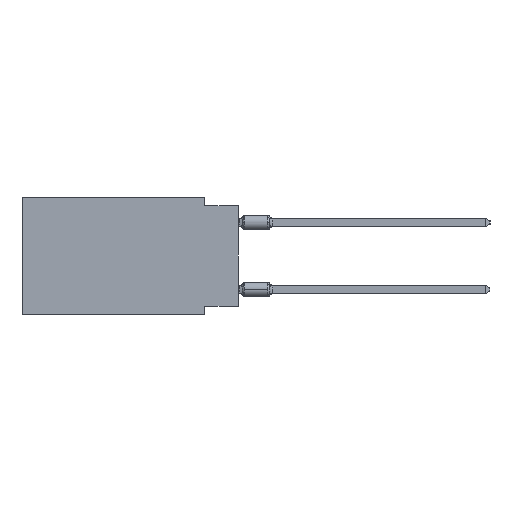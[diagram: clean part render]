
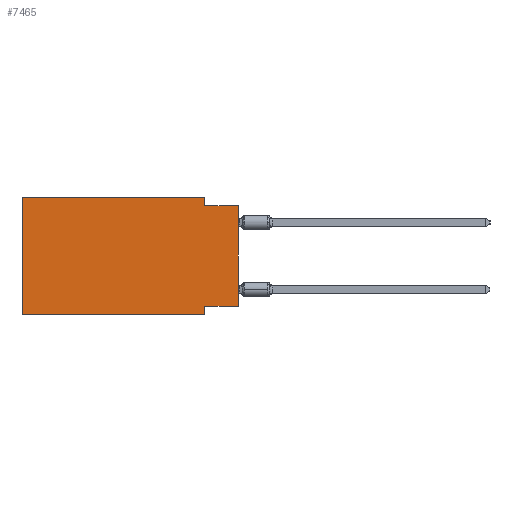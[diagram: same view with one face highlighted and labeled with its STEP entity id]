
A CAD part, left-side view. The second image highlights one B-rep face of the part: STEP entity #7465.
In plain terms, the highlighted planar face has unit normal (-1, 0, 0).
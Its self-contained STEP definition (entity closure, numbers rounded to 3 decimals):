
#809 = DIRECTION ( 'NONE',  ( 0., 0., -1. ) ) ;
#2652 = LINE ( 'NONE', #35970, #9058 ) ;
#2998 = VECTOR ( 'NONE', #25973, 1000. ) ;
#3244 = ORIENTED_EDGE ( 'NONE', *, *, #29201, .F. ) ;
#3809 = DIRECTION ( 'NONE',  ( 0., 1., 0. ) ) ;
#4959 = CARTESIAN_POINT ( 'NONE',  ( 0., 16.383, 0. ) ) ;
#5069 = FACE_OUTER_BOUND ( 'NONE', #7067, .T. ) ;
#5259 = LINE ( 'NONE', #28649, #10199 ) ;
#6622 = EDGE_CURVE ( 'NONE', #28197, #38506, #11860, .T. ) ;
#7067 = EDGE_LOOP ( 'NONE', ( #33655, #41532, #22445, #38807, #16646, #17941, #14594, #3244 ) ) ;
#7431 = AXIS2_PLACEMENT_3D ( 'NONE', #24636, #37595, #8459 ) ;
#7465 = ADVANCED_FACE ( 'NONE', ( #5069 ), #11648, .F. ) ;
#8037 = CARTESIAN_POINT ( 'NONE',  ( 0., 16.383, 0. ) ) ;
#8459 = DIRECTION ( 'NONE',  ( 0., 0., -1. ) ) ;
#8770 = EDGE_CURVE ( 'NONE', #38506, #9479, #41892, .T. ) ;
#9046 = DIRECTION ( 'NONE',  ( 0., -1., 0. ) ) ;
#9058 = VECTOR ( 'NONE', #38172, 1000. ) ;
#9479 = VERTEX_POINT ( 'NONE', #29926 ) ;
#10199 = VECTOR ( 'NONE', #15889, 1000. ) ;
#11470 = EDGE_CURVE ( 'NONE', #16207, #28123, #5259, .T. ) ;
#11648 = PLANE ( 'NONE',  #7431 ) ;
#11763 = VERTEX_POINT ( 'NONE', #16727 ) ;
#11860 = LINE ( 'NONE', #8037, #12814 ) ;
#12764 = CARTESIAN_POINT ( 'NONE',  ( 0., 16.383, 0. ) ) ;
#12814 = VECTOR ( 'NONE', #30595, 1000. ) ;
#12991 = LINE ( 'NONE', #22785, #2998 ) ;
#13105 = EDGE_CURVE ( 'NONE', #28197, #16300, #37562, .T. ) ;
#13923 = VECTOR ( 'NONE', #809, 1000. ) ;
#14243 = EDGE_CURVE ( 'NONE', #35062, #28123, #12991, .T. ) ;
#14594 = ORIENTED_EDGE ( 'NONE', *, *, #15758, .F. ) ;
#15758 = EDGE_CURVE ( 'NONE', #11763, #16300, #2652, .T. ) ;
#15889 = DIRECTION ( 'NONE',  ( 0., -1., 0. ) ) ;
#16207 = VERTEX_POINT ( 'NONE', #26573 ) ;
#16300 = VERTEX_POINT ( 'NONE', #36765 ) ;
#16646 = ORIENTED_EDGE ( 'NONE', *, *, #6622, .F. ) ;
#16727 = CARTESIAN_POINT ( 'NONE',  ( 0., 2.54, -8.255 ) ) ;
#17914 = VECTOR ( 'NONE', #9046, 1000. ) ;
#17941 = ORIENTED_EDGE ( 'NONE', *, *, #13105, .T. ) ;
#19251 = VECTOR ( 'NONE', #3809, 1000. ) ;
#22445 = ORIENTED_EDGE ( 'NONE', *, *, #23297, .F. ) ;
#22785 = CARTESIAN_POINT ( 'NONE',  ( 0., 0., 0. ) ) ;
#23297 = EDGE_CURVE ( 'NONE', #9479, #16207, #32961, .T. ) ;
#23388 = CARTESIAN_POINT ( 'NONE',  ( 0., 2.54, 0. ) ) ;
#24191 = VECTOR ( 'NONE', #25744, 1000. ) ;
#24636 = CARTESIAN_POINT ( 'NONE',  ( 0., 16.383, 0. ) ) ;
#25744 = DIRECTION ( 'NONE',  ( 0., -1., 0. ) ) ;
#25973 = DIRECTION ( 'NONE',  ( 0., 0., 1. ) ) ;
#26468 = CARTESIAN_POINT ( 'NONE',  ( 0., 0., -0.635 ) ) ;
#26573 = CARTESIAN_POINT ( 'NONE',  ( 0., 2.54, -0.635 ) ) ;
#28123 = VERTEX_POINT ( 'NONE', #26468 ) ;
#28197 = VERTEX_POINT ( 'NONE', #37088 ) ;
#28649 = CARTESIAN_POINT ( 'NONE',  ( 0., 0., -0.635 ) ) ;
#29201 = EDGE_CURVE ( 'NONE', #35062, #11763, #35922, .T. ) ;
#29926 = CARTESIAN_POINT ( 'NONE',  ( 0., 2.54, 0. ) ) ;
#30595 = DIRECTION ( 'NONE',  ( 0., 0., 1. ) ) ;
#31593 = CARTESIAN_POINT ( 'NONE',  ( 0., 16.383, -8.89 ) ) ;
#31771 = CARTESIAN_POINT ( 'NONE',  ( 0., 0., -8.255 ) ) ;
#32959 = CARTESIAN_POINT ( 'NONE',  ( 0., 0., -8.255 ) ) ;
#32961 = LINE ( 'NONE', #23388, #13923 ) ;
#33655 = ORIENTED_EDGE ( 'NONE', *, *, #14243, .T. ) ;
#35062 = VERTEX_POINT ( 'NONE', #31771 ) ;
#35922 = LINE ( 'NONE', #32959, #19251 ) ;
#35970 = CARTESIAN_POINT ( 'NONE',  ( 0., 2.54, -8.89 ) ) ;
#36765 = CARTESIAN_POINT ( 'NONE',  ( 0., 2.54, -8.89 ) ) ;
#37088 = CARTESIAN_POINT ( 'NONE',  ( 0., 16.383, -8.89 ) ) ;
#37562 = LINE ( 'NONE', #31593, #17914 ) ;
#37595 = DIRECTION ( 'NONE',  ( 1., 0., 0. ) ) ;
#38172 = DIRECTION ( 'NONE',  ( 0., 0., -1. ) ) ;
#38506 = VERTEX_POINT ( 'NONE', #4959 ) ;
#38807 = ORIENTED_EDGE ( 'NONE', *, *, #8770, .F. ) ;
#41532 = ORIENTED_EDGE ( 'NONE', *, *, #11470, .F. ) ;
#41892 = LINE ( 'NONE', #12764, #24191 ) ;
